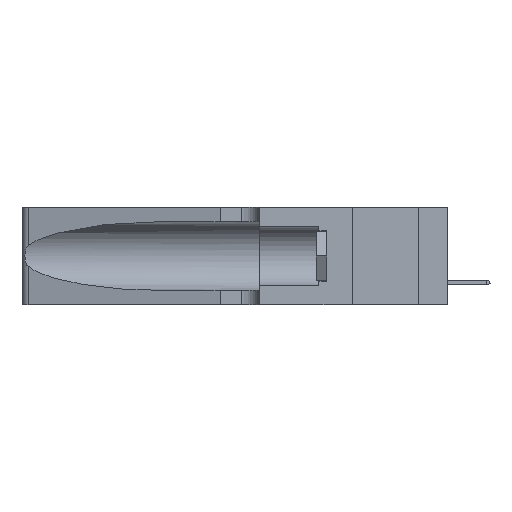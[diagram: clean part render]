
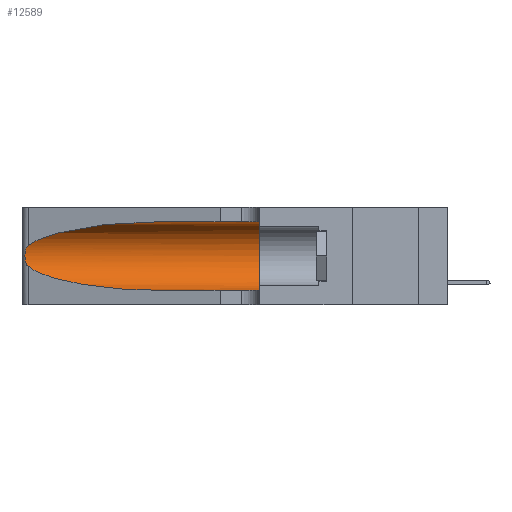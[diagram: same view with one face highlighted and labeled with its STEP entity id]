
A CAD part, left-side view. The second image highlights one B-rep face of the part: STEP entity #12589.
In plain terms, the highlighted cylindrical face has radius 3.308 mm (diameter 6.617 mm), a partial arc.
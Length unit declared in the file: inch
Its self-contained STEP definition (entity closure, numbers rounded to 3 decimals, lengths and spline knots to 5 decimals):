
#1487 = DIRECTION ( 'NONE',  ( 0., 1., 0. ) ) ;
#2753 = CARTESIAN_POINT ( 'NONE',  ( 0.25787, 1.23484, 0.2124 ) ) ;
#3076 = CARTESIAN_POINT ( 'NONE',  ( 0.25854, 1.2359, 0.20912 ) ) ;
#3207 = VERTEX_POINT ( 'NONE', #17875 ) ;
#3242 = CARTESIAN_POINT ( 'NONE',  ( 0.18966, 0.96281, 0.05475 ) ) ;
#3547 = VERTEX_POINT ( 'NONE', #39086 ) ;
#4130 = EDGE_CURVE ( 'NONE', #42716, #40701, #37213, .T. ) ;
#4374 = AXIS2_PLACEMENT_3D ( 'NONE', #20078, #1487, #37875 ) ;
#4796 = CIRCLE ( 'NONE', #4374, 0.13025 ) ;
#5772 = VERTEX_POINT ( 'NONE', #21083 ) ;
#5999 = VECTOR ( 'NONE', #12112, 39.37008 ) ;
#6261 = CARTESIAN_POINT ( 'NONE',  ( 0.25487, 1.22718, 0.22369 ) ) ;
#6886 = CARTESIAN_POINT ( 'NONE',  ( 0.26075, 1.23896, 0.19203 ) ) ;
#6961 = CARTESIAN_POINT ( 'NONE',  ( 0.1305, 1.61858, 0.185 ) ) ;
#7299 = AXIS2_PLACEMENT_3D ( 'NONE', #6961, #14428, #43439 ) ;
#7504 = EDGE_CURVE ( 'NONE', #3207, #33441, #34920, .T. ) ;
#12112 = DIRECTION ( 'NONE',  ( 0., -1., 0. ) ) ;
#12271 = EDGE_LOOP ( 'NONE', ( #40745, #26755, #32423, #30739, #28721, #31294 ) ) ;
#12589 = ADVANCED_FACE ( 'NONE', ( #37983 ), #45279, .F. ) ;
#13726 = CARTESIAN_POINT ( 'NONE',  ( 0.25487, 1.22718, 0.14631 ) ) ;
#14428 = DIRECTION ( 'NONE',  ( 0., -1., 0. ) ) ;
#17215 = CARTESIAN_POINT ( 'NONE',  ( 0.25555, 1.22993, 0.14849 ) ) ;
#17693 = CARTESIAN_POINT ( 'NONE',  ( 0.2373, 1.15595, 0.08982 ) ) ;
#17875 = CARTESIAN_POINT ( 'NONE',  ( 0.25487, 1.22718, 0.22369 ) ) ;
#18726 = CARTESIAN_POINT ( 'NONE',  ( 0.18966, 0.96281, 0.31525 ) ) ;
#18977 = EDGE_CURVE ( 'NONE', #5772, #3547, #27738, .T. ) ;
#19280 = CARTESIAN_POINT ( 'NONE',  ( 0.1305, 1.61858, 0.05475 ) ) ;
#19537 = DIRECTION ( 'NONE',  ( 0., -1., 0. ) ) ;
#20078 = CARTESIAN_POINT ( 'NONE',  ( 0.1305, 0.35, 0.185 ) ) ;
#20195 = CARTESIAN_POINT ( 'NONE',  ( 0.1305, 1.61858, 0.31525 ) ) ;
#21083 = CARTESIAN_POINT ( 'NONE',  ( 0.1305, 0.72297, 0.31525 ) ) ;
#21340 = CARTESIAN_POINT ( 'NONE',  ( 0.26018, 1.23835, 0.19895 ) ) ;
#21480 = CARTESIAN_POINT ( 'NONE',  ( 0.25789, 1.23486, 0.15765 ) ) ;
#23857 = CARTESIAN_POINT ( 'NONE',  ( 0.25639, 1.23184, 0.21858 ) ) ;
#24513 = CARTESIAN_POINT ( 'NONE',  ( 0.25856, 1.23593, 0.16098 ) ) ;
#25031 = CARTESIAN_POINT ( 'NONE',  ( 0.25487, 1.22718, 0.14631 ) ) ;
#25116 = CARTESIAN_POINT ( 'NONE',  ( 0.25639, 1.23186, 0.15144 ) ) ;
#25438 = CARTESIAN_POINT ( 'NONE',  ( 0.1305, 0.72297, 0.05475 ) ) ;
#26755 = ORIENTED_EDGE ( 'NONE', *, *, #7504, .T. ) ;
#27008 =( BOUNDED_CURVE ( )  B_SPLINE_CURVE ( 3, ( #39614, #18726, #46507, #39463 ),
 .UNSPECIFIED., .F., .F. ) 
 B_SPLINE_CURVE_WITH_KNOTS ( ( 4, 4 ),
 ( 1.5708, 2.84003 ),
 .UNSPECIFIED. ) 
 CURVE ( )  GEOMETRIC_REPRESENTATION_ITEM ( )  RATIONAL_B_SPLINE_CURVE ( ( 1., 0.87, 0.87, 1. ) ) 
 REPRESENTATION_ITEM ( '' )  );
#27738 = LINE ( 'NONE', #20195, #43589 ) ;
#28341 = CARTESIAN_POINT ( 'NONE',  ( 0.25487, 1.22718, 0.14631 ) ) ;
#28673 = CARTESIAN_POINT ( 'NONE',  ( 0.1305, 0.72297, 0.05475 ) ) ;
#28721 = ORIENTED_EDGE ( 'NONE', *, *, #31656, .F. ) ;
#30739 = ORIENTED_EDGE ( 'NONE', *, *, #4130, .T. ) ;
#31294 = ORIENTED_EDGE ( 'NONE', *, *, #18977, .F. ) ;
#31656 = EDGE_CURVE ( 'NONE', #3547, #40701, #4796, .T. ) ;
#32292 = CARTESIAN_POINT ( 'NONE',  ( 0.26075, 1.23896, 0.178 ) ) ;
#32423 = ORIENTED_EDGE ( 'NONE', *, *, #32786, .T. ) ;
#32786 = EDGE_CURVE ( 'NONE', #33441, #42716, #40406, .T. ) ;
#33441 = VERTEX_POINT ( 'NONE', #25031 ) ;
#34920 = B_SPLINE_CURVE_WITH_KNOTS ( 'NONE', 3,
 ( #6261, #35316, #23857, #2753, #3076, #21340, #6886, #32292, #43207, #24513, #21480, #25116, #17215, #13726 ),
 .UNSPECIFIED., .F., .F.,
 ( 4, 2, 2, 2, 2, 2, 4 ),
 ( 0., 0.00027, 0.00053, 0.00107, 0.0016, 0.00187, 0.00214 ),
 .UNSPECIFIED. ) ;
#35316 = CARTESIAN_POINT ( 'NONE',  ( 0.25555, 1.22994, 0.2215 ) ) ;
#37213 = LINE ( 'NONE', #19280, #5999 ) ;
#37875 = DIRECTION ( 'NONE',  ( 0., 0., 1. ) ) ;
#37983 = FACE_OUTER_BOUND ( 'NONE', #12271, .T. ) ;
#39086 = CARTESIAN_POINT ( 'NONE',  ( 0.1305, 0.35, 0.31525 ) ) ;
#39463 = CARTESIAN_POINT ( 'NONE',  ( 0.25487, 1.22718, 0.22369 ) ) ;
#39614 = CARTESIAN_POINT ( 'NONE',  ( 0.1305, 0.72297, 0.31525 ) ) ;
#40406 =( BOUNDED_CURVE ( )  B_SPLINE_CURVE ( 3, ( #28341, #17693, #3242, #28673 ),
 .UNSPECIFIED., .F., .T. ) 
 B_SPLINE_CURVE_WITH_KNOTS ( ( 4, 4 ),
 ( 3.44316, 4.71239 ),
 .UNSPECIFIED. ) 
 CURVE ( )  GEOMETRIC_REPRESENTATION_ITEM ( )  RATIONAL_B_SPLINE_CURVE ( ( 1., 0.87, 0.87, 1. ) ) 
 REPRESENTATION_ITEM ( '' )  );
#40596 = EDGE_CURVE ( 'NONE', #5772, #3207, #27008, .T. ) ;
#40701 = VERTEX_POINT ( 'NONE', #41128 ) ;
#40745 = ORIENTED_EDGE ( 'NONE', *, *, #40596, .T. ) ;
#41128 = CARTESIAN_POINT ( 'NONE',  ( 0.1305, 0.35, 0.05475 ) ) ;
#42716 = VERTEX_POINT ( 'NONE', #25438 ) ;
#43207 = CARTESIAN_POINT ( 'NONE',  ( 0.26017, 1.23833, 0.17102 ) ) ;
#43439 = DIRECTION ( 'NONE',  ( 0., 0., -1. ) ) ;
#43589 = VECTOR ( 'NONE', #19537, 39.37008 ) ;
#45279 = CYLINDRICAL_SURFACE ( 'NONE', #7299, 0.13025 ) ;
#46507 = CARTESIAN_POINT ( 'NONE',  ( 0.2373, 1.15595, 0.28018 ) ) ;
